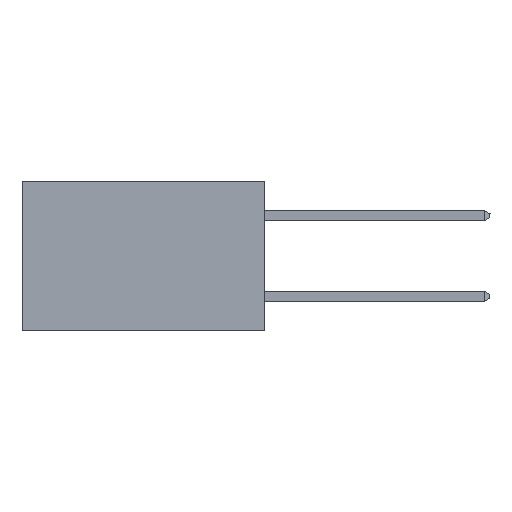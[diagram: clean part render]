
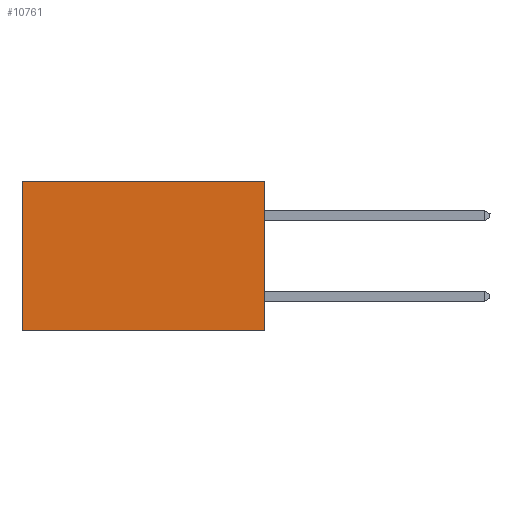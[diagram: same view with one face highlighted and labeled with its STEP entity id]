
A CAD part, left-side view. The second image highlights one B-rep face of the part: STEP entity #10761.
In plain terms, the highlighted planar face has unit normal (-1, 0, 0).
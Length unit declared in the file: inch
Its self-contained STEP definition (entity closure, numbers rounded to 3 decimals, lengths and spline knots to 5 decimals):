
#1684 = VECTOR ( 'NONE', #24374, 39.37008 ) ;
#1691 = CARTESIAN_POINT ( 'NONE',  ( 0.298, 0., -0.37 ) ) ;
#1986 = DIRECTION ( 'NONE',  ( 0., 0., -1. ) ) ;
#2098 = CARTESIAN_POINT ( 'NONE',  ( 0.298, 0., 0. ) ) ;
#3665 = VERTEX_POINT ( 'NONE', #31949 ) ;
#4069 = CARTESIAN_POINT ( 'NONE',  ( 0.298, 0.6, 0. ) ) ;
#6378 = ORIENTED_EDGE ( 'NONE', *, *, #26951, .T. ) ;
#6473 = FACE_OUTER_BOUND ( 'NONE', #30173, .T. ) ;
#7200 = CARTESIAN_POINT ( 'NONE',  ( 0.298, 0., 0. ) ) ;
#8037 = CARTESIAN_POINT ( 'NONE',  ( 0.298, 0.6, -0.37 ) ) ;
#9269 = AXIS2_PLACEMENT_3D ( 'NONE', #2098, #29402, #1986 ) ;
#9496 = DIRECTION ( 'NONE',  ( 0., 1., 0. ) ) ;
#9501 = ORIENTED_EDGE ( 'NONE', *, *, #21223, .F. ) ;
#10045 = VERTEX_POINT ( 'NONE', #8037 ) ;
#10761 = ADVANCED_FACE ( 'NONE', ( #6473 ), #26770, .F. ) ;
#10976 = CARTESIAN_POINT ( 'NONE',  ( 0.298, 0., -0.37 ) ) ;
#11059 = CARTESIAN_POINT ( 'NONE',  ( 0.298, 0.6, 0. ) ) ;
#11291 = VERTEX_POINT ( 'NONE', #4069 ) ;
#12822 = ORIENTED_EDGE ( 'NONE', *, *, #26358, .T. ) ;
#13547 = VECTOR ( 'NONE', #9496, 39.37008 ) ;
#13957 = ORIENTED_EDGE ( 'NONE', *, *, #24872, .F. ) ;
#17818 = VECTOR ( 'NONE', #23745, 39.37008 ) ;
#20793 = LINE ( 'NONE', #25126, #1684 ) ;
#21223 = EDGE_CURVE ( 'NONE', #29470, #10045, #26451, .T. ) ;
#23745 = DIRECTION ( 'NONE',  ( 0., 0., -1. ) ) ;
#24133 = VECTOR ( 'NONE', #29239, 39.37008 ) ;
#24374 = DIRECTION ( 'NONE',  ( 0., 0., -1. ) ) ;
#24872 = EDGE_CURVE ( 'NONE', #3665, #29470, #20793, .T. ) ;
#25126 = CARTESIAN_POINT ( 'NONE',  ( 0.298, 0., 0. ) ) ;
#26358 = EDGE_CURVE ( 'NONE', #3665, #11291, #29910, .T. ) ;
#26451 = LINE ( 'NONE', #1691, #24133 ) ;
#26770 = PLANE ( 'NONE',  #9269 ) ;
#26951 = EDGE_CURVE ( 'NONE', #11291, #10045, #27511, .T. ) ;
#27511 = LINE ( 'NONE', #11059, #17818 ) ;
#29239 = DIRECTION ( 'NONE',  ( 0., 1., 0. ) ) ;
#29402 = DIRECTION ( 'NONE',  ( 1., 0., 0. ) ) ;
#29470 = VERTEX_POINT ( 'NONE', #10976 ) ;
#29910 = LINE ( 'NONE', #7200, #13547 ) ;
#30173 = EDGE_LOOP ( 'NONE', ( #6378, #9501, #13957, #12822 ) ) ;
#31949 = CARTESIAN_POINT ( 'NONE',  ( 0.298, 0., 0. ) ) ;
